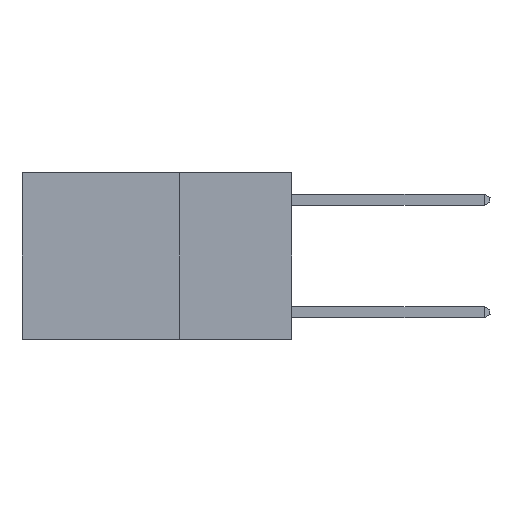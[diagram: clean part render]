
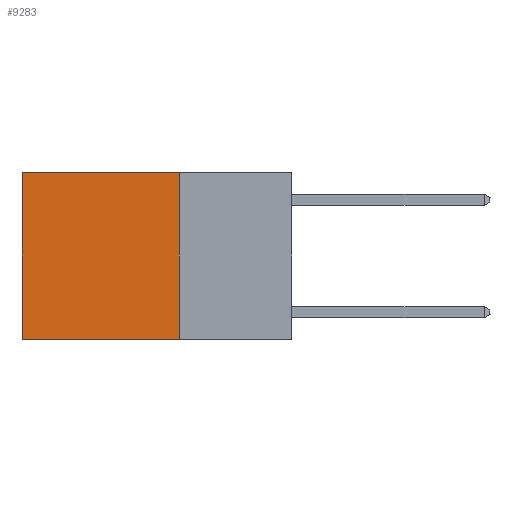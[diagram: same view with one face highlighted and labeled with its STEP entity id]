
A CAD part, left-side view. The second image highlights one B-rep face of the part: STEP entity #9283.
In plain terms, the highlighted planar face has unit normal (-1, 0, 0).
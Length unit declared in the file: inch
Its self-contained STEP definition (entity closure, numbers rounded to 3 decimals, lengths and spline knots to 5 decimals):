
#243 = AXIS2_PLACEMENT_3D ( 'NONE', #968, #786, #848 ) ;
#420 = VECTOR ( 'NONE', #11797, 39.37008 ) ;
#423 = VERTEX_POINT ( 'NONE', #7462 ) ;
#786 = DIRECTION ( 'NONE',  ( 1., 0., 0. ) ) ;
#848 = DIRECTION ( 'NONE',  ( 0., 0., -1. ) ) ;
#968 = CARTESIAN_POINT ( 'NONE',  ( 0.2625, 0.25, 0. ) ) ;
#983 = CARTESIAN_POINT ( 'NONE',  ( 0.2625, 0.6, 0. ) ) ;
#999 = DIRECTION ( 'NONE',  ( 0., 0., -1. ) ) ;
#1692 = FACE_OUTER_BOUND ( 'NONE', #11028, .T. ) ;
#1882 = CARTESIAN_POINT ( 'NONE',  ( 0.2625, 0.25, -0.37 ) ) ;
#2283 = LINE ( 'NONE', #11613, #420 ) ;
#2599 = CARTESIAN_POINT ( 'NONE',  ( 0.2625, 0.6, -0.37 ) ) ;
#2888 = ORIENTED_EDGE ( 'NONE', *, *, #9299, .F. ) ;
#3493 = EDGE_CURVE ( 'NONE', #4515, #7583, #2283, .T. ) ;
#3620 = EDGE_CURVE ( 'NONE', #4515, #423, #9253, .T. ) ;
#4196 = EDGE_CURVE ( 'NONE', #7583, #6178, #10245, .T. ) ;
#4411 = CARTESIAN_POINT ( 'NONE',  ( 0.2625, 0.25, 0. ) ) ;
#4515 = VERTEX_POINT ( 'NONE', #4411 ) ;
#5499 = VECTOR ( 'NONE', #999, 39.37008 ) ;
#6178 = VERTEX_POINT ( 'NONE', #2599 ) ;
#7250 = VECTOR ( 'NONE', #11196, 39.37008 ) ;
#7462 = CARTESIAN_POINT ( 'NONE',  ( 0.2625, 0.25, -0.37 ) ) ;
#7583 = VERTEX_POINT ( 'NONE', #983 ) ;
#8288 = DIRECTION ( 'NONE',  ( 0., 0., -1. ) ) ;
#8399 = CARTESIAN_POINT ( 'NONE',  ( 0.2625, 0.25, 0. ) ) ;
#8992 = VECTOR ( 'NONE', #8288, 39.37008 ) ;
#9133 = PLANE ( 'NONE',  #243 ) ;
#9253 = LINE ( 'NONE', #8399, #8992 ) ;
#9283 = ADVANCED_FACE ( 'NONE', ( #1692 ), #9133, .F. ) ;
#9299 = EDGE_CURVE ( 'NONE', #423, #6178, #10220, .T. ) ;
#9353 = CARTESIAN_POINT ( 'NONE',  ( 0.2625, 0.6, 0. ) ) ;
#10220 = LINE ( 'NONE', #1882, #7250 ) ;
#10245 = LINE ( 'NONE', #9353, #5499 ) ;
#10472 = ORIENTED_EDGE ( 'NONE', *, *, #3493, .T. ) ;
#11028 = EDGE_LOOP ( 'NONE', ( #11840, #2888, #11229, #10472 ) ) ;
#11196 = DIRECTION ( 'NONE',  ( 0., 1., 0. ) ) ;
#11229 = ORIENTED_EDGE ( 'NONE', *, *, #3620, .F. ) ;
#11613 = CARTESIAN_POINT ( 'NONE',  ( 0.2625, 0.25, 0. ) ) ;
#11797 = DIRECTION ( 'NONE',  ( 0., 1., 0. ) ) ;
#11840 = ORIENTED_EDGE ( 'NONE', *, *, #4196, .T. ) ;
